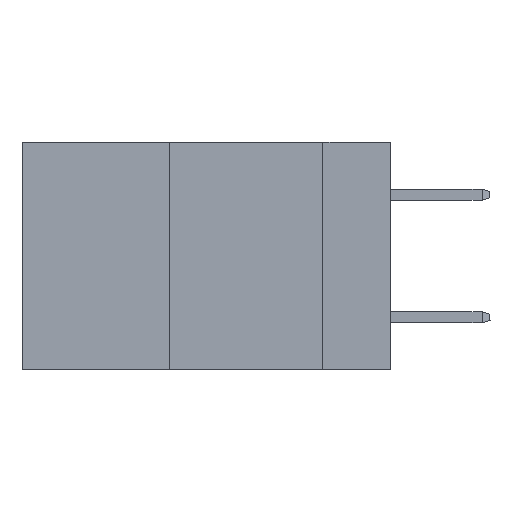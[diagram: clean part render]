
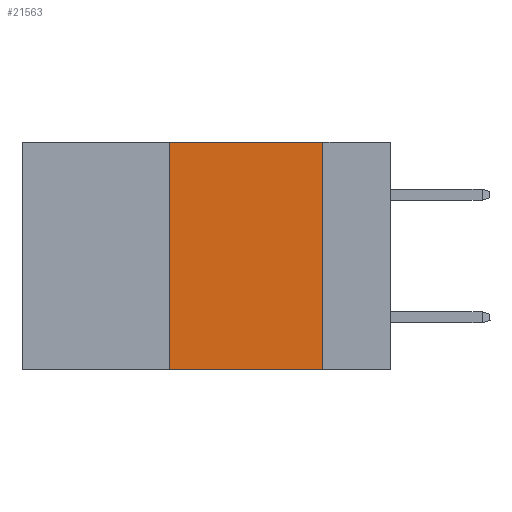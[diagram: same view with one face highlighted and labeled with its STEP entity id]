
A CAD part, left-side view. The second image highlights one B-rep face of the part: STEP entity #21563.
In plain terms, the highlighted planar face has unit normal (-1, 0, 0).
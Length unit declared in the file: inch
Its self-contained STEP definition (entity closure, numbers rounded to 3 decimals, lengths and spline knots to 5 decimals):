
#1370 = CARTESIAN_POINT ( 'NONE',  ( 0., 0.6, 0. ) ) ;
#2506 = CARTESIAN_POINT ( 'NONE',  ( 0., 0.11, -0.37 ) ) ;
#3577 = AXIS2_PLACEMENT_3D ( 'NONE', #1370, #4095, #4198 ) ;
#3905 = CARTESIAN_POINT ( 'NONE',  ( 0., 0.11, 0. ) ) ;
#3937 = ORIENTED_EDGE ( 'NONE', *, *, #26711, .F. ) ;
#4095 = DIRECTION ( 'NONE',  ( 1., 0., 0. ) ) ;
#4198 = DIRECTION ( 'NONE',  ( 0., 0., -1. ) ) ;
#5652 = LINE ( 'NONE', #14386, #23037 ) ;
#6177 = CARTESIAN_POINT ( 'NONE',  ( 0., 0.36, 0. ) ) ;
#6358 = EDGE_CURVE ( 'NONE', #24735, #17694, #17771, .T. ) ;
#6730 = VERTEX_POINT ( 'NONE', #33021 ) ;
#8367 = EDGE_CURVE ( 'NONE', #6730, #17694, #23868, .T. ) ;
#10043 = DIRECTION ( 'NONE',  ( 0., -1., 0. ) ) ;
#12033 = DIRECTION ( 'NONE',  ( 0., 0., 1. ) ) ;
#12698 = VECTOR ( 'NONE', #28096, 39.37008 ) ;
#13298 = EDGE_CURVE ( 'NONE', #27265, #24735, #30613, .T. ) ;
#14194 = EDGE_LOOP ( 'NONE', ( #25644, #30903, #3937, #17522 ) ) ;
#14386 = CARTESIAN_POINT ( 'NONE',  ( 0., 0.36, 0. ) ) ;
#16995 = CARTESIAN_POINT ( 'NONE',  ( 0., 0.6, -0.37 ) ) ;
#17522 = ORIENTED_EDGE ( 'NONE', *, *, #8367, .T. ) ;
#17694 = VERTEX_POINT ( 'NONE', #2506 ) ;
#17771 = LINE ( 'NONE', #3905, #12698 ) ;
#19711 = DIRECTION ( 'NONE',  ( 0., -1., 0. ) ) ;
#19935 = PLANE ( 'NONE',  #3577 ) ;
#21563 = ADVANCED_FACE ( 'NONE', ( #30343 ), #19935, .F. ) ;
#21758 = CARTESIAN_POINT ( 'NONE',  ( 0., 0.11, 0. ) ) ;
#23037 = VECTOR ( 'NONE', #12033, 39.37008 ) ;
#23868 = LINE ( 'NONE', #16995, #31498 ) ;
#24735 = VERTEX_POINT ( 'NONE', #21758 ) ;
#25644 = ORIENTED_EDGE ( 'NONE', *, *, #6358, .F. ) ;
#26711 = EDGE_CURVE ( 'NONE', #6730, #27265, #5652, .T. ) ;
#27141 = VECTOR ( 'NONE', #10043, 39.37008 ) ;
#27265 = VERTEX_POINT ( 'NONE', #6177 ) ;
#28096 = DIRECTION ( 'NONE',  ( 0., 0., -1. ) ) ;
#28817 = CARTESIAN_POINT ( 'NONE',  ( 0., 0.6, 0. ) ) ;
#30343 = FACE_OUTER_BOUND ( 'NONE', #14194, .T. ) ;
#30613 = LINE ( 'NONE', #28817, #27141 ) ;
#30903 = ORIENTED_EDGE ( 'NONE', *, *, #13298, .F. ) ;
#31498 = VECTOR ( 'NONE', #19711, 39.37008 ) ;
#33021 = CARTESIAN_POINT ( 'NONE',  ( 0., 0.36, -0.37 ) ) ;
